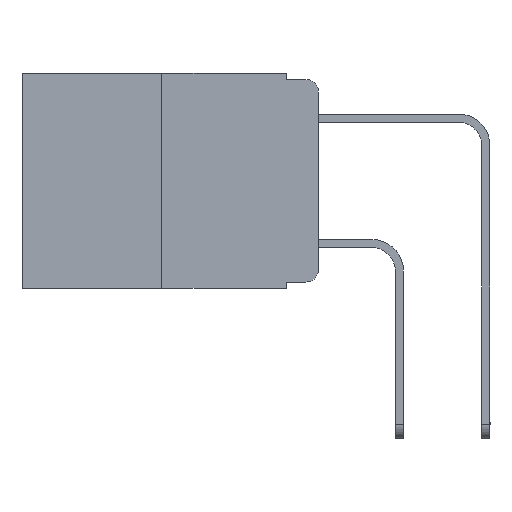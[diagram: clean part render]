
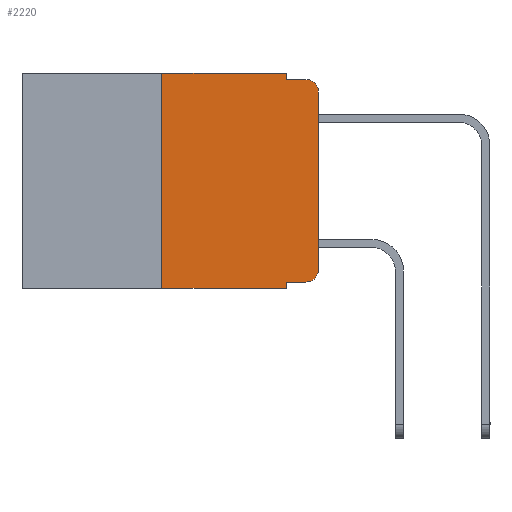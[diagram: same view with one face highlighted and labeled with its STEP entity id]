
A CAD part, left-side view. The second image highlights one B-rep face of the part: STEP entity #2220.
In plain terms, the highlighted planar face has unit normal (-1, 0, 0).
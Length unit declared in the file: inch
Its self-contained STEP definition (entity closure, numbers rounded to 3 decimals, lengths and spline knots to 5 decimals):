
#336 = AXIS2_PLACEMENT_3D ( 'NONE', #10026, #12282, #10953 ) ;
#406 = DIRECTION ( 'NONE',  ( 0., 0., -1. ) ) ;
#464 = EDGE_CURVE ( 'NONE', #11721, #9460, #1757, .T. ) ;
#519 = CARTESIAN_POINT ( 'NONE',  ( 0., 0., -0.313 ) ) ;
#719 = DIRECTION ( 'NONE',  ( 0., -1., 0. ) ) ;
#1014 = EDGE_CURVE ( 'NONE', #1298, #11269, #8877, .T. ) ;
#1032 = DIRECTION ( 'NONE',  ( 0., 0., 1. ) ) ;
#1298 = VERTEX_POINT ( 'NONE', #11970 ) ;
#1757 = CIRCLE ( 'NONE', #12143, 0.02 ) ;
#1760 = LINE ( 'NONE', #4086, #3872 ) ;
#1777 = CARTESIAN_POINT ( 'NONE',  ( 0., 0.051, -0.333 ) ) ;
#1900 = VECTOR ( 'NONE', #13391, 39.37008 ) ;
#1995 = EDGE_CURVE ( 'NONE', #8980, #12819, #11360, .T. ) ;
#2015 = ORIENTED_EDGE ( 'NONE', *, *, #5317, .T. ) ;
#2051 = CARTESIAN_POINT ( 'NONE',  ( 0., 0.02, -0.03 ) ) ;
#2086 = CARTESIAN_POINT ( 'NONE',  ( 0., 0.051, 0. ) ) ;
#2220 = ADVANCED_FACE ( 'NONE', ( #2463 ), #9824, .F. ) ;
#2330 = DIRECTION ( 'NONE',  ( 1., 0., 0. ) ) ;
#2463 = FACE_OUTER_BOUND ( 'NONE', #12260, .T. ) ;
#2482 = CARTESIAN_POINT ( 'NONE',  ( 0., 0.051, -0.333 ) ) ;
#2577 = DIRECTION ( 'NONE',  ( 0., 0., -1. ) ) ;
#2679 = CARTESIAN_POINT ( 'NONE',  ( 0., 0.051, -0.01 ) ) ;
#2836 = DIRECTION ( 'NONE',  ( 0., -1., 0. ) ) ;
#2966 = CARTESIAN_POINT ( 'NONE',  ( 0., 0.02, -0.333 ) ) ;
#3000 = CARTESIAN_POINT ( 'NONE',  ( 0., 0.25, -0.343 ) ) ;
#3010 = CARTESIAN_POINT ( 'NONE',  ( 0., 0., 0. ) ) ;
#3203 = DIRECTION ( 'NONE',  ( -1., 0., 0. ) ) ;
#3253 = EDGE_CURVE ( 'NONE', #12159, #9887, #4943, .T. ) ;
#3501 = VERTEX_POINT ( 'NONE', #5294 ) ;
#3504 = CIRCLE ( 'NONE', #336, 0.02 ) ;
#3872 = VECTOR ( 'NONE', #2836, 39.37008 ) ;
#4086 = CARTESIAN_POINT ( 'NONE',  ( 0., 0.473, -0.343 ) ) ;
#4316 = CARTESIAN_POINT ( 'NONE',  ( 0., 0.02, -0.01 ) ) ;
#4572 = ORIENTED_EDGE ( 'NONE', *, *, #7368, .F. ) ;
#4643 = AXIS2_PLACEMENT_3D ( 'NONE', #13059, #2330, #406 ) ;
#4851 = DIRECTION ( 'NONE',  ( 0., 0., 1. ) ) ;
#4943 = LINE ( 'NONE', #1777, #7560 ) ;
#5096 = ORIENTED_EDGE ( 'NONE', *, *, #1995, .F. ) ;
#5178 = LINE ( 'NONE', #3010, #8928 ) ;
#5294 = CARTESIAN_POINT ( 'NONE',  ( 0., 0.051, -0.343 ) ) ;
#5317 = EDGE_CURVE ( 'NONE', #9887, #13212, #3504, .T. ) ;
#5428 = EDGE_CURVE ( 'NONE', #11269, #9460, #8336, .T. ) ;
#5451 = ORIENTED_EDGE ( 'NONE', *, *, #11099, .T. ) ;
#6043 = CARTESIAN_POINT ( 'NONE',  ( 0., 0.25, 0. ) ) ;
#6099 = EDGE_CURVE ( 'NONE', #13212, #11721, #5178, .T. ) ;
#6187 = DIRECTION ( 'NONE',  ( 0., -1., 0. ) ) ;
#6503 = CARTESIAN_POINT ( 'NONE',  ( 0., 0.051, -0.01 ) ) ;
#6781 = VECTOR ( 'NONE', #4851, 39.37008 ) ;
#7169 = VECTOR ( 'NONE', #6187, 39.37008 ) ;
#7368 = EDGE_CURVE ( 'NONE', #12159, #3501, #9582, .T. ) ;
#7369 = ORIENTED_EDGE ( 'NONE', *, *, #5428, .F. ) ;
#7560 = VECTOR ( 'NONE', #719, 39.37008 ) ;
#7689 = ORIENTED_EDGE ( 'NONE', *, *, #6099, .T. ) ;
#8054 = LINE ( 'NONE', #10167, #7169 ) ;
#8336 = LINE ( 'NONE', #2679, #1900 ) ;
#8568 = EDGE_CURVE ( 'NONE', #12819, #1298, #8054, .T. ) ;
#8877 = LINE ( 'NONE', #10067, #11706 ) ;
#8928 = VECTOR ( 'NONE', #1032, 39.37008 ) ;
#8955 = VECTOR ( 'NONE', #10727, 39.37008 ) ;
#8980 = VERTEX_POINT ( 'NONE', #3000 ) ;
#9460 = VERTEX_POINT ( 'NONE', #4316 ) ;
#9582 = LINE ( 'NONE', #2086, #8955 ) ;
#9824 = PLANE ( 'NONE',  #4643 ) ;
#9887 = VERTEX_POINT ( 'NONE', #2966 ) ;
#10026 = CARTESIAN_POINT ( 'NONE',  ( 0., 0.02, -0.313 ) ) ;
#10056 = CARTESIAN_POINT ( 'NONE',  ( 0., 0., -0.03 ) ) ;
#10067 = CARTESIAN_POINT ( 'NONE',  ( 0., 0.051, 0. ) ) ;
#10167 = CARTESIAN_POINT ( 'NONE',  ( 0., 0.473, 0. ) ) ;
#10693 = DIRECTION ( 'NONE',  ( 0., 0., -1. ) ) ;
#10727 = DIRECTION ( 'NONE',  ( 0., 0., -1. ) ) ;
#10779 = ORIENTED_EDGE ( 'NONE', *, *, #8568, .F. ) ;
#10953 = DIRECTION ( 'NONE',  ( 0., 0., -1. ) ) ;
#11099 = EDGE_CURVE ( 'NONE', #8980, #3501, #1760, .T. ) ;
#11269 = VERTEX_POINT ( 'NONE', #6503 ) ;
#11360 = LINE ( 'NONE', #13467, #6781 ) ;
#11706 = VECTOR ( 'NONE', #2577, 39.37008 ) ;
#11721 = VERTEX_POINT ( 'NONE', #10056 ) ;
#11970 = CARTESIAN_POINT ( 'NONE',  ( 0., 0.051, 0. ) ) ;
#12143 = AXIS2_PLACEMENT_3D ( 'NONE', #2051, #3203, #10693 ) ;
#12149 = ORIENTED_EDGE ( 'NONE', *, *, #3253, .T. ) ;
#12159 = VERTEX_POINT ( 'NONE', #2482 ) ;
#12260 = EDGE_LOOP ( 'NONE', ( #7689, #12483, #7369, #13478, #10779, #5096, #5451, #4572, #12149, #2015 ) ) ;
#12282 = DIRECTION ( 'NONE',  ( -1., 0., 0. ) ) ;
#12483 = ORIENTED_EDGE ( 'NONE', *, *, #464, .T. ) ;
#12819 = VERTEX_POINT ( 'NONE', #6043 ) ;
#13059 = CARTESIAN_POINT ( 'NONE',  ( 0., 0.473, 0. ) ) ;
#13212 = VERTEX_POINT ( 'NONE', #519 ) ;
#13391 = DIRECTION ( 'NONE',  ( 0., -1., 0. ) ) ;
#13467 = CARTESIAN_POINT ( 'NONE',  ( 0., 0.25, 0. ) ) ;
#13478 = ORIENTED_EDGE ( 'NONE', *, *, #1014, .F. ) ;
